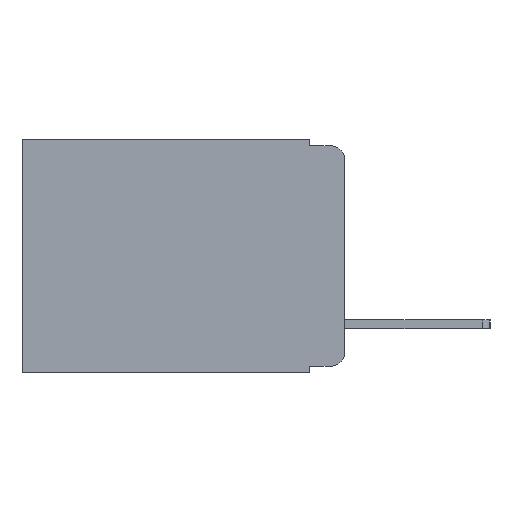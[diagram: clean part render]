
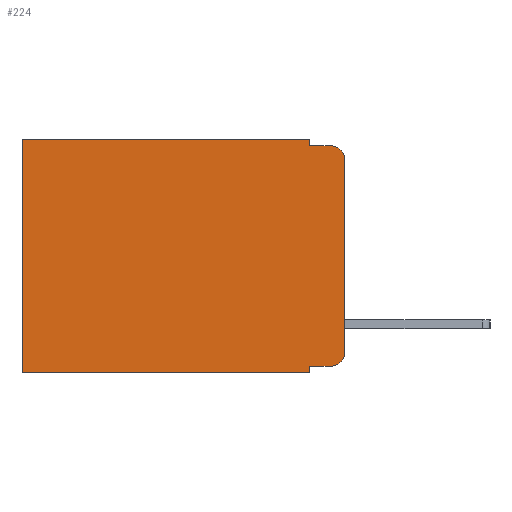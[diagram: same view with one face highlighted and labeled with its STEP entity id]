
A CAD part, left-side view. The second image highlights one B-rep face of the part: STEP entity #224.
In plain terms, the highlighted planar face has unit normal (-1, 0, 0).
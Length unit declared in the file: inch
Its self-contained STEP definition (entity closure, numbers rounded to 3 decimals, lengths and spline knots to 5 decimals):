
#159 = ORIENTED_EDGE ( 'NONE', *, *, #16280, .F. ) ;
#224 = ADVANCED_FACE ( 'NONE', ( #6767 ), #9326, .F. ) ;
#890 = VECTOR ( 'NONE', #17088, 39.37008 ) ;
#980 = ORIENTED_EDGE ( 'NONE', *, *, #15359, .T. ) ;
#1104 = VECTOR ( 'NONE', #10738, 39.37008 ) ;
#1178 = VERTEX_POINT ( 'NONE', #17565 ) ;
#1226 = CARTESIAN_POINT ( 'NONE',  ( 0.298, 0.051, 0. ) ) ;
#1412 = EDGE_CURVE ( 'NONE', #4892, #5098, #1572, .T. ) ;
#1433 = LINE ( 'NONE', #14706, #13047 ) ;
#1532 = VECTOR ( 'NONE', #10679, 39.37008 ) ;
#1572 = LINE ( 'NONE', #1226, #1104 ) ;
#1886 = LINE ( 'NONE', #4277, #12634 ) ;
#2843 = CARTESIAN_POINT ( 'NONE',  ( 0.298, 0.051, -0.01 ) ) ;
#3064 = CARTESIAN_POINT ( 'NONE',  ( 0.298, 0.473, 0. ) ) ;
#3071 = ORIENTED_EDGE ( 'NONE', *, *, #10289, .F. ) ;
#3095 = ORIENTED_EDGE ( 'NONE', *, *, #6281, .F. ) ;
#3127 = ORIENTED_EDGE ( 'NONE', *, *, #13224, .T. ) ;
#3184 = ORIENTED_EDGE ( 'NONE', *, *, #1412, .F. ) ;
#3557 = ORIENTED_EDGE ( 'NONE', *, *, #16535, .F. ) ;
#3884 = VERTEX_POINT ( 'NONE', #9293 ) ;
#4029 = LINE ( 'NONE', #2843, #7838 ) ;
#4277 = CARTESIAN_POINT ( 'NONE',  ( 0.298, 0.473, 0. ) ) ;
#4414 = LINE ( 'NONE', #9159, #890 ) ;
#4714 = CARTESIAN_POINT ( 'NONE',  ( 0.298, 0.051, 0. ) ) ;
#4892 = VERTEX_POINT ( 'NONE', #4714 ) ;
#5098 = VERTEX_POINT ( 'NONE', #13335 ) ;
#5327 = DIRECTION ( 'NONE',  ( 0., 0., -1. ) ) ;
#5413 = DIRECTION ( 'NONE',  ( -1., 0., 0. ) ) ;
#5424 = LINE ( 'NONE', #7096, #12204 ) ;
#5547 = CIRCLE ( 'NONE', #17675, 0.02 ) ;
#5731 = VERTEX_POINT ( 'NONE', #12407 ) ;
#6011 = VERTEX_POINT ( 'NONE', #16833 ) ;
#6279 = ORIENTED_EDGE ( 'NONE', *, *, #17304, .T. ) ;
#6281 = EDGE_CURVE ( 'NONE', #6011, #5731, #1433, .T. ) ;
#6361 = CARTESIAN_POINT ( 'NONE',  ( 0.298, 0.02, -0.333 ) ) ;
#6740 = ORIENTED_EDGE ( 'NONE', *, *, #7792, .T. ) ;
#6767 = FACE_OUTER_BOUND ( 'NONE', #14912, .T. ) ;
#6815 = CARTESIAN_POINT ( 'NONE',  ( 0.298, 0.02, -0.313 ) ) ;
#7096 = CARTESIAN_POINT ( 'NONE',  ( 0.298, 0., 0. ) ) ;
#7299 = ORIENTED_EDGE ( 'NONE', *, *, #10317, .T. ) ;
#7792 = EDGE_CURVE ( 'NONE', #6011, #11487, #17861, .T. ) ;
#7838 = VECTOR ( 'NONE', #8544, 39.37008 ) ;
#8130 = DIRECTION ( 'NONE',  ( 0., 0., -1. ) ) ;
#8477 = DIRECTION ( 'NONE',  ( 0., 1., 0. ) ) ;
#8544 = DIRECTION ( 'NONE',  ( 0., -1., 0. ) ) ;
#8889 = VERTEX_POINT ( 'NONE', #3064 ) ;
#9159 = CARTESIAN_POINT ( 'NONE',  ( 0.298, 0.051, -0.333 ) ) ;
#9293 = CARTESIAN_POINT ( 'NONE',  ( 0.298, 0.473, -0.343 ) ) ;
#9326 = PLANE ( 'NONE',  #16808 ) ;
#9352 = DIRECTION ( 'NONE',  ( 1., 0., 0. ) ) ;
#9357 = CARTESIAN_POINT ( 'NONE',  ( 0.298, 0.051, 0. ) ) ;
#9381 = DIRECTION ( 'NONE',  ( 0., 0., -1. ) ) ;
#10289 = EDGE_CURVE ( 'NONE', #17027, #1178, #12732, .T. ) ;
#10317 = EDGE_CURVE ( 'NONE', #12328, #5731, #5547, .T. ) ;
#10679 = DIRECTION ( 'NONE',  ( 0., 0., -1. ) ) ;
#10730 = CARTESIAN_POINT ( 'NONE',  ( 0.298, 0., 0. ) ) ;
#10738 = DIRECTION ( 'NONE',  ( 0., 0., -1. ) ) ;
#11145 = AXIS2_PLACEMENT_3D ( 'NONE', #13481, #5413, #14782 ) ;
#11487 = VERTEX_POINT ( 'NONE', #13708 ) ;
#12030 = CARTESIAN_POINT ( 'NONE',  ( 0.298, 0., -0.343 ) ) ;
#12040 = VECTOR ( 'NONE', #13344, 39.37008 ) ;
#12204 = VECTOR ( 'NONE', #8477, 39.37008 ) ;
#12328 = VERTEX_POINT ( 'NONE', #6361 ) ;
#12407 = CARTESIAN_POINT ( 'NONE',  ( 0.298, 0., -0.313 ) ) ;
#12463 = LINE ( 'NONE', #12030, #12040 ) ;
#12634 = VECTOR ( 'NONE', #17742, 39.37008 ) ;
#12732 = LINE ( 'NONE', #9357, #1532 ) ;
#13047 = VECTOR ( 'NONE', #5327, 39.37008 ) ;
#13224 = EDGE_CURVE ( 'NONE', #4892, #8889, #5424, .T. ) ;
#13335 = CARTESIAN_POINT ( 'NONE',  ( 0.298, 0.051, -0.01 ) ) ;
#13344 = DIRECTION ( 'NONE',  ( 0., 1., 0. ) ) ;
#13481 = CARTESIAN_POINT ( 'NONE',  ( 0.298, 0.02, -0.03 ) ) ;
#13708 = CARTESIAN_POINT ( 'NONE',  ( 0.298, 0.02, -0.01 ) ) ;
#14558 = CARTESIAN_POINT ( 'NONE',  ( 0.298, 0.051, -0.333 ) ) ;
#14706 = CARTESIAN_POINT ( 'NONE',  ( 0.298, 0., 0. ) ) ;
#14782 = DIRECTION ( 'NONE',  ( 0., 0., -1. ) ) ;
#14912 = EDGE_LOOP ( 'NONE', ( #3095, #6740, #3557, #3184, #3127, #6279, #159, #3071, #980, #7299 ) ) ;
#15359 = EDGE_CURVE ( 'NONE', #17027, #12328, #4414, .T. ) ;
#16069 = DIRECTION ( 'NONE',  ( -1., 0., 0. ) ) ;
#16280 = EDGE_CURVE ( 'NONE', #1178, #3884, #12463, .T. ) ;
#16535 = EDGE_CURVE ( 'NONE', #5098, #11487, #4029, .T. ) ;
#16808 = AXIS2_PLACEMENT_3D ( 'NONE', #10730, #9352, #9381 ) ;
#16833 = CARTESIAN_POINT ( 'NONE',  ( 0.298, 0., -0.03 ) ) ;
#17027 = VERTEX_POINT ( 'NONE', #14558 ) ;
#17088 = DIRECTION ( 'NONE',  ( 0., -1., 0. ) ) ;
#17304 = EDGE_CURVE ( 'NONE', #8889, #3884, #1886, .T. ) ;
#17565 = CARTESIAN_POINT ( 'NONE',  ( 0.298, 0.051, -0.343 ) ) ;
#17675 = AXIS2_PLACEMENT_3D ( 'NONE', #6815, #16069, #8130 ) ;
#17742 = DIRECTION ( 'NONE',  ( 0., 0., -1. ) ) ;
#17861 = CIRCLE ( 'NONE', #11145, 0.02 ) ;
